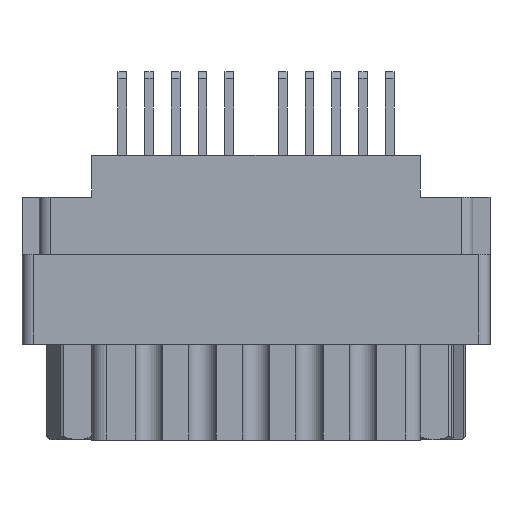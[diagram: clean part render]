
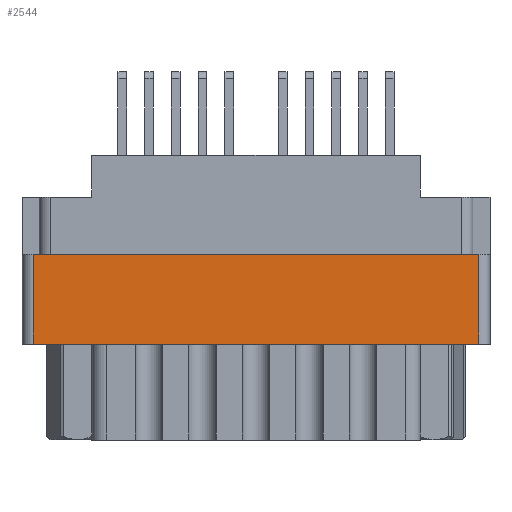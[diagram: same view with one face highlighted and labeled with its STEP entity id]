
A CAD part, front view. The second image highlights one B-rep face of the part: STEP entity #2544.
In plain terms, the highlighted planar face has unit normal (0, -1, 0).
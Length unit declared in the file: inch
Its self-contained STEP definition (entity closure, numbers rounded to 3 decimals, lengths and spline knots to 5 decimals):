
#500 = EDGE_LOOP ( 'NONE', ( #36990, #976, #7163, #28036 ) ) ;
#880 = CARTESIAN_POINT ( 'NONE',  ( 0.624, -0.343, -0.529 ) ) ;
#976 = ORIENTED_EDGE ( 'NONE', *, *, #8366, .T. ) ;
#1152 = AXIS2_PLACEMENT_3D ( 'NONE', #13472, #24926, #22109 ) ;
#1900 = CARTESIAN_POINT ( 'NONE',  ( 0.624, -0.343, -0.798 ) ) ;
#2544 = ADVANCED_FACE ( 'NONE', ( #36576 ), #7806, .T. ) ;
#3794 = VECTOR ( 'NONE', #5092, 39.37008 ) ;
#4085 = VERTEX_POINT ( 'NONE', #24931 ) ;
#4611 = DIRECTION ( 'NONE',  ( 1., 0., 0. ) ) ;
#5092 = DIRECTION ( 'NONE',  ( 0., 0., 1. ) ) ;
#6143 = VECTOR ( 'NONE', #34015, 39.37008 ) ;
#7163 = ORIENTED_EDGE ( 'NONE', *, *, #30529, .F. ) ;
#7442 = LINE ( 'NONE', #21550, #22647 ) ;
#7806 = PLANE ( 'NONE',  #1152 ) ;
#8366 = EDGE_CURVE ( 'NONE', #17534, #4085, #7442, .T. ) ;
#9573 = CARTESIAN_POINT ( 'NONE',  ( 0.624, -0.343, -0.277 ) ) ;
#10371 = LINE ( 'NONE', #1900, #3794 ) ;
#12742 = VERTEX_POINT ( 'NONE', #9573 ) ;
#13472 = CARTESIAN_POINT ( 'NONE',  ( -0.656, -0.343, -0.798 ) ) ;
#15174 = VECTOR ( 'NONE', #4611, 39.37008 ) ;
#16025 = VERTEX_POINT ( 'NONE', #880 ) ;
#17062 = CARTESIAN_POINT ( 'NONE',  ( 0., -0.343, -0.529 ) ) ;
#17534 = VERTEX_POINT ( 'NONE', #24043 ) ;
#21550 = CARTESIAN_POINT ( 'NONE',  ( -0.624, -0.343, -0.798 ) ) ;
#21926 = DIRECTION ( 'NONE',  ( 0., 0., -1. ) ) ;
#22109 = DIRECTION ( 'NONE',  ( 0., 0., -1. ) ) ;
#22647 = VECTOR ( 'NONE', #21926, 39.37008 ) ;
#23957 = EDGE_CURVE ( 'NONE', #17534, #12742, #30561, .T. ) ;
#24043 = CARTESIAN_POINT ( 'NONE',  ( -0.624, -0.343, -0.277 ) ) ;
#24926 = DIRECTION ( 'NONE',  ( 0., -1., 0. ) ) ;
#24931 = CARTESIAN_POINT ( 'NONE',  ( -0.624, -0.343, -0.529 ) ) ;
#26092 = LINE ( 'NONE', #17062, #6143 ) ;
#28036 = ORIENTED_EDGE ( 'NONE', *, *, #31394, .T. ) ;
#30529 = EDGE_CURVE ( 'NONE', #16025, #4085, #26092, .T. ) ;
#30561 = LINE ( 'NONE', #30928, #15174 ) ;
#30928 = CARTESIAN_POINT ( 'NONE',  ( 0., -0.343, -0.277 ) ) ;
#31394 = EDGE_CURVE ( 'NONE', #16025, #12742, #10371, .T. ) ;
#34015 = DIRECTION ( 'NONE',  ( -1., 0., 0. ) ) ;
#36576 = FACE_OUTER_BOUND ( 'NONE', #500, .T. ) ;
#36990 = ORIENTED_EDGE ( 'NONE', *, *, #23957, .F. ) ;
